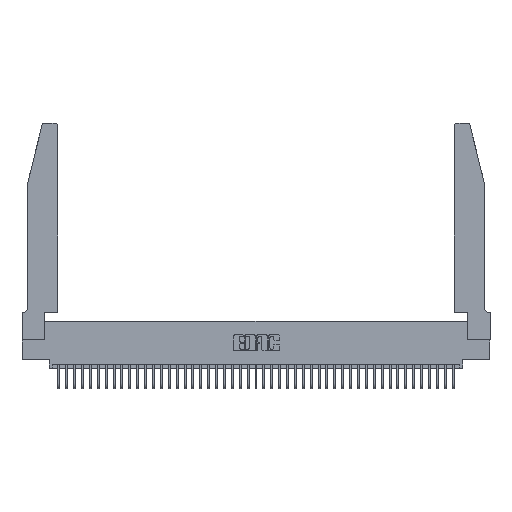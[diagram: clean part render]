
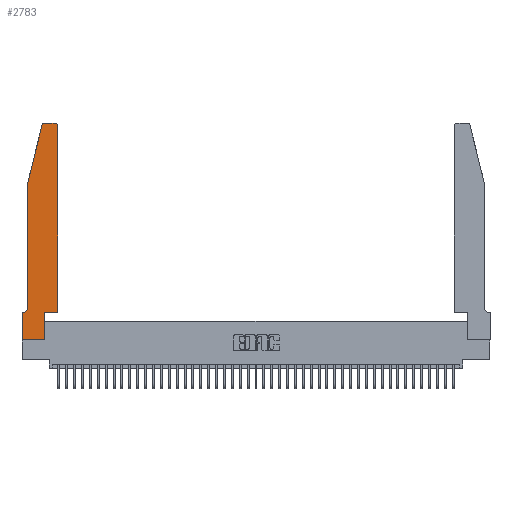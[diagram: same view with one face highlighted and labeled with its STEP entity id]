
A CAD part, top view. The second image highlights one B-rep face of the part: STEP entity #2783.
In plain terms, the highlighted planar face has unit normal (0, 0, 1).
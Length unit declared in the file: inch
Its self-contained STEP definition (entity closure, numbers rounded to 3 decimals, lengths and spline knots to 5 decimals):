
#482 = CARTESIAN_POINT ( 'NONE',  ( 0.284, 2.72, 0.37 ) ) ;
#603 = VECTOR ( 'NONE', #15723, 39.37008 ) ;
#744 = DIRECTION ( 'NONE',  ( -1., 0., 0. ) ) ;
#1351 = CARTESIAN_POINT ( 'NONE',  ( 0.0055, 0.42, 0.37 ) ) ;
#1936 = CARTESIAN_POINT ( 'NONE',  ( 0., 0.35, 0.37 ) ) ;
#1998 = CARTESIAN_POINT ( 'NONE',  ( 0., 0., 0.37 ) ) ;
#2783 = ADVANCED_FACE ( 'NONE', ( #6500 ), #26719, .T. ) ;
#3357 = VECTOR ( 'NONE', #744, 39.37008 ) ;
#3570 = EDGE_CURVE ( 'NONE', #15780, #8260, #39818, .T. ) ;
#4051 = DIRECTION ( 'NONE',  ( 1., 0., 0. ) ) ;
#4730 = DIRECTION ( 'NONE',  ( 1., 0., 0. ) ) ;
#4887 = VERTEX_POINT ( 'NONE', #20597 ) ;
#4920 = DIRECTION ( 'NONE',  ( -1., 0., 0. ) ) ;
#5535 = ORIENTED_EDGE ( 'NONE', *, *, #15825, .T. ) ;
#5649 = CARTESIAN_POINT ( 'NONE',  ( 0., 0.35, 0.37 ) ) ;
#5687 = CIRCLE ( 'NONE', #6532, 0.03 ) ;
#6343 = ORIENTED_EDGE ( 'NONE', *, *, #10176, .T. ) ;
#6500 = FACE_OUTER_BOUND ( 'NONE', #25654, .T. ) ;
#6532 = AXIS2_PLACEMENT_3D ( 'NONE', #16802, #41146, #20307 ) ;
#7408 = ORIENTED_EDGE ( 'NONE', *, *, #32376, .T. ) ;
#7500 = LINE ( 'NONE', #11420, #43548 ) ;
#8100 = EDGE_CURVE ( 'NONE', #13126, #35681, #7500, .T. ) ;
#8260 = VERTEX_POINT ( 'NONE', #43394 ) ;
#8404 = ORIENTED_EDGE ( 'NONE', *, *, #10188, .T. ) ;
#8961 = VECTOR ( 'NONE', #19393, 39.37008 ) ;
#9232 = DIRECTION ( 'NONE',  ( 0., 0., 1. ) ) ;
#10082 = LINE ( 'NONE', #26076, #603 ) ;
#10176 = EDGE_CURVE ( 'NONE', #13020, #41701, #10082, .T. ) ;
#10188 = EDGE_CURVE ( 'NONE', #4887, #15780, #28741, .T. ) ;
#10284 = VECTOR ( 'NONE', #4730, 39.37008 ) ;
#11068 = DIRECTION ( 'NONE',  ( 0., 1., 0. ) ) ;
#11413 = LINE ( 'NONE', #22342, #10284 ) ;
#11420 = CARTESIAN_POINT ( 'NONE',  ( 0.0755, 2., 0.37 ) ) ;
#11666 = CARTESIAN_POINT ( 'NONE',  ( 0.2865, 0., 0.37 ) ) ;
#11804 = ORIENTED_EDGE ( 'NONE', *, *, #45293, .T. ) ;
#12871 = CARTESIAN_POINT ( 'NONE',  ( 0.4505, 0.35, 0.37 ) ) ;
#13020 = VERTEX_POINT ( 'NONE', #12871 ) ;
#13126 = VERTEX_POINT ( 'NONE', #20500 ) ;
#14040 = CARTESIAN_POINT ( 'NONE',  ( 0.284, 2.75, 0.37 ) ) ;
#14892 = VECTOR ( 'NONE', #26636, 39.37008 ) ;
#15286 = CARTESIAN_POINT ( 'NONE',  ( 0.0755, 2., 0.37 ) ) ;
#15675 = CARTESIAN_POINT ( 'NONE',  ( 0.4505, 2.72, 0.37 ) ) ;
#15721 = CARTESIAN_POINT ( 'NONE',  ( 0.0755, 0.42, 0.37 ) ) ;
#15723 = DIRECTION ( 'NONE',  ( 0., 1., 0. ) ) ;
#15780 = VERTEX_POINT ( 'NONE', #11666 ) ;
#15825 = EDGE_CURVE ( 'NONE', #35795, #30261, #16695, .T. ) ;
#16048 = ORIENTED_EDGE ( 'NONE', *, *, #25154, .T. ) ;
#16695 = CIRCLE ( 'NONE', #18494, 0.07 ) ;
#16802 = CARTESIAN_POINT ( 'NONE',  ( 0.4205, 2.72, 0.37 ) ) ;
#16848 = ORIENTED_EDGE ( 'NONE', *, *, #26915, .T. ) ;
#18494 = AXIS2_PLACEMENT_3D ( 'NONE', #1351, #25992, #4920 ) ;
#19393 = DIRECTION ( 'NONE',  ( 1., 0., 0. ) ) ;
#20068 = VERTEX_POINT ( 'NONE', #1936 ) ;
#20307 = DIRECTION ( 'NONE',  ( 1., 0., 0. ) ) ;
#20500 = CARTESIAN_POINT ( 'NONE',  ( 0.25487, 2.72718, 0.37 ) ) ;
#20597 = CARTESIAN_POINT ( 'NONE',  ( 0., 0., 0.37 ) ) ;
#21808 = ORIENTED_EDGE ( 'NONE', *, *, #36525, .T. ) ;
#22241 = EDGE_CURVE ( 'NONE', #35681, #35795, #33824, .T. ) ;
#22342 = CARTESIAN_POINT ( 'NONE',  ( 0.4505, 0.35, 0.37 ) ) ;
#24552 = VECTOR ( 'NONE', #35420, 39.37008 ) ;
#25149 = DIRECTION ( 'NONE',  ( 0., 0., 1. ) ) ;
#25154 = EDGE_CURVE ( 'NONE', #30261, #20068, #28814, .T. ) ;
#25654 = EDGE_LOOP ( 'NONE', ( #16848, #43363, #36659, #37296, #5535, #16048, #21808, #8404, #40374, #7408, #6343, #11804 ) ) ;
#25992 = DIRECTION ( 'NONE',  ( 0., 0., -1. ) ) ;
#26076 = CARTESIAN_POINT ( 'NONE',  ( 0.4505, 0.35, 0.37 ) ) ;
#26636 = DIRECTION ( 'NONE',  ( 0., -1., 0. ) ) ;
#26719 = PLANE ( 'NONE',  #36055 ) ;
#26915 = EDGE_CURVE ( 'NONE', #32329, #35429, #31411, .T. ) ;
#27707 = VECTOR ( 'NONE', #40389, 39.37008 ) ;
#28200 = CARTESIAN_POINT ( 'NONE',  ( 0.0055, 0.35, 0.37 ) ) ;
#28323 = EDGE_CURVE ( 'NONE', #35429, #13126, #32388, .T. ) ;
#28517 = CARTESIAN_POINT ( 'NONE',  ( 0.2865, 0.35, 0.37 ) ) ;
#28741 = LINE ( 'NONE', #40205, #8961 ) ;
#28814 = LINE ( 'NONE', #29948, #27707 ) ;
#29361 = CARTESIAN_POINT ( 'NONE',  ( 0.4205, 2.75, 0.37 ) ) ;
#29948 = CARTESIAN_POINT ( 'NONE',  ( 0.0755, 0.35, 0.37 ) ) ;
#30261 = VERTEX_POINT ( 'NONE', #28200 ) ;
#31411 = LINE ( 'NONE', #42740, #3357 ) ;
#31848 = CARTESIAN_POINT ( 'NONE',  ( 0.0755, 2., 0.37 ) ) ;
#32329 = VERTEX_POINT ( 'NONE', #29361 ) ;
#32335 = LINE ( 'NONE', #1998, #14892 ) ;
#32376 = EDGE_CURVE ( 'NONE', #8260, #13020, #11413, .T. ) ;
#32388 = CIRCLE ( 'NONE', #37733, 0.03 ) ;
#33713 = DIRECTION ( 'NONE',  ( 1., 0., 0. ) ) ;
#33824 = LINE ( 'NONE', #31848, #24552 ) ;
#35420 = DIRECTION ( 'NONE',  ( 0., -1., 0. ) ) ;
#35429 = VERTEX_POINT ( 'NONE', #14040 ) ;
#35681 = VERTEX_POINT ( 'NONE', #15286 ) ;
#35786 = DIRECTION ( 'NONE',  ( -0.239, -0.971, 0. ) ) ;
#35795 = VERTEX_POINT ( 'NONE', #15721 ) ;
#36055 = AXIS2_PLACEMENT_3D ( 'NONE', #5649, #9232, #33713 ) ;
#36525 = EDGE_CURVE ( 'NONE', #20068, #4887, #32335, .T. ) ;
#36659 = ORIENTED_EDGE ( 'NONE', *, *, #8100, .T. ) ;
#37296 = ORIENTED_EDGE ( 'NONE', *, *, #22241, .T. ) ;
#37733 = AXIS2_PLACEMENT_3D ( 'NONE', #482, #25149, #4051 ) ;
#39818 = LINE ( 'NONE', #28517, #40889 ) ;
#40205 = CARTESIAN_POINT ( 'NONE',  ( 0., 0., 0.37 ) ) ;
#40374 = ORIENTED_EDGE ( 'NONE', *, *, #3570, .T. ) ;
#40389 = DIRECTION ( 'NONE',  ( -1., 0., 0. ) ) ;
#40889 = VECTOR ( 'NONE', #11068, 39.37008 ) ;
#41146 = DIRECTION ( 'NONE',  ( 0., 0., 1. ) ) ;
#41701 = VERTEX_POINT ( 'NONE', #15675 ) ;
#42740 = CARTESIAN_POINT ( 'NONE',  ( 0.2605, 2.75, 0.37 ) ) ;
#43363 = ORIENTED_EDGE ( 'NONE', *, *, #28323, .T. ) ;
#43394 = CARTESIAN_POINT ( 'NONE',  ( 0.2865, 0.35, 0.37 ) ) ;
#43548 = VECTOR ( 'NONE', #35786, 39.37008 ) ;
#45293 = EDGE_CURVE ( 'NONE', #41701, #32329, #5687, .T. ) ;
